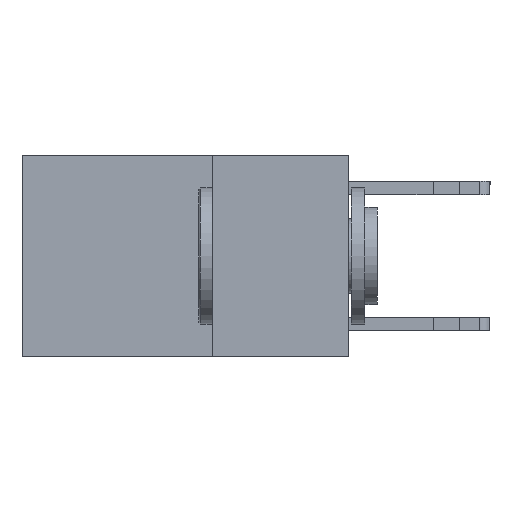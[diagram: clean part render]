
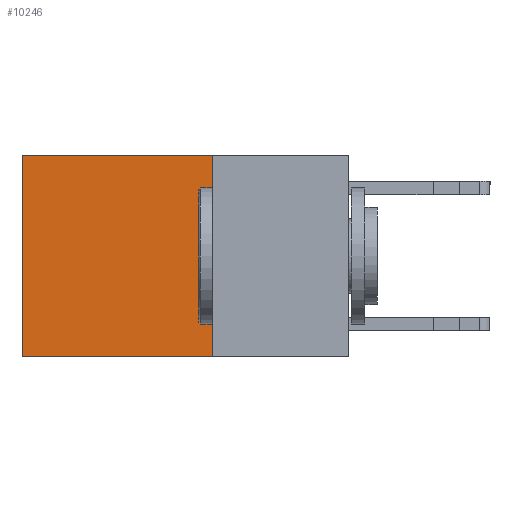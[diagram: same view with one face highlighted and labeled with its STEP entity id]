
A CAD part, left-side view. The second image highlights one B-rep face of the part: STEP entity #10246.
In plain terms, the highlighted planar face has unit normal (-1, 0, 0).
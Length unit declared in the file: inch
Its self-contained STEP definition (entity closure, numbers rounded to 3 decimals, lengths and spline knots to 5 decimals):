
#128 = EDGE_CURVE ( 'NONE', #10606, #3293, #6848, .T. ) ;
#142 = CARTESIAN_POINT ( 'NONE',  ( 0.2625, 0.25, 0. ) ) ;
#1308 = CARTESIAN_POINT ( 'NONE',  ( 0.2625, 0.25, 0. ) ) ;
#1750 = ORIENTED_EDGE ( 'NONE', *, *, #4822, .T. ) ;
#2732 = DIRECTION ( 'NONE',  ( 0., 0., -1. ) ) ;
#3293 = VERTEX_POINT ( 'NONE', #4863 ) ;
#3451 = FACE_OUTER_BOUND ( 'NONE', #6504, .T. ) ;
#3484 = ORIENTED_EDGE ( 'NONE', *, *, #3889, .F. ) ;
#3889 = EDGE_CURVE ( 'NONE', #3293, #4288, #6079, .T. ) ;
#4245 = VERTEX_POINT ( 'NONE', #9427 ) ;
#4288 = VERTEX_POINT ( 'NONE', #10548 ) ;
#4417 = CARTESIAN_POINT ( 'NONE',  ( 0.2625, 0.25, 0. ) ) ;
#4525 = AXIS2_PLACEMENT_3D ( 'NONE', #1308, #7777, #5625 ) ;
#4576 = PLANE ( 'NONE',  #4525 ) ;
#4822 = EDGE_CURVE ( 'NONE', #4245, #4288, #12455, .T. ) ;
#4863 = CARTESIAN_POINT ( 'NONE',  ( 0.2625, 0.25, -0.37 ) ) ;
#5223 = DIRECTION ( 'NONE',  ( 0., 1., 0. ) ) ;
#5291 = VECTOR ( 'NONE', #9141, 39.37008 ) ;
#5443 = EDGE_CURVE ( 'NONE', #10606, #4245, #7808, .T. ) ;
#5625 = DIRECTION ( 'NONE',  ( 0., 0., -1. ) ) ;
#5670 = ORIENTED_EDGE ( 'NONE', *, *, #128, .F. ) ;
#6079 = LINE ( 'NONE', #11752, #9572 ) ;
#6504 = EDGE_LOOP ( 'NONE', ( #1750, #3484, #5670, #12477 ) ) ;
#6601 = DIRECTION ( 'NONE',  ( 0., 1., 0. ) ) ;
#6848 = LINE ( 'NONE', #7913, #5291 ) ;
#7777 = DIRECTION ( 'NONE',  ( 1., 0., 0. ) ) ;
#7808 = LINE ( 'NONE', #142, #11655 ) ;
#7913 = CARTESIAN_POINT ( 'NONE',  ( 0.2625, 0.25, 0. ) ) ;
#8267 = CARTESIAN_POINT ( 'NONE',  ( 0.2625, 0.6, 0. ) ) ;
#9141 = DIRECTION ( 'NONE',  ( 0., 0., -1. ) ) ;
#9427 = CARTESIAN_POINT ( 'NONE',  ( 0.2625, 0.6, 0. ) ) ;
#9572 = VECTOR ( 'NONE', #5223, 39.37008 ) ;
#10246 = ADVANCED_FACE ( 'NONE', ( #3451 ), #4576, .F. ) ;
#10548 = CARTESIAN_POINT ( 'NONE',  ( 0.2625, 0.6, -0.37 ) ) ;
#10606 = VERTEX_POINT ( 'NONE', #4417 ) ;
#11655 = VECTOR ( 'NONE', #6601, 39.37008 ) ;
#11752 = CARTESIAN_POINT ( 'NONE',  ( 0.2625, 0.25, -0.37 ) ) ;
#11861 = VECTOR ( 'NONE', #2732, 39.37008 ) ;
#12455 = LINE ( 'NONE', #8267, #11861 ) ;
#12477 = ORIENTED_EDGE ( 'NONE', *, *, #5443, .T. ) ;
